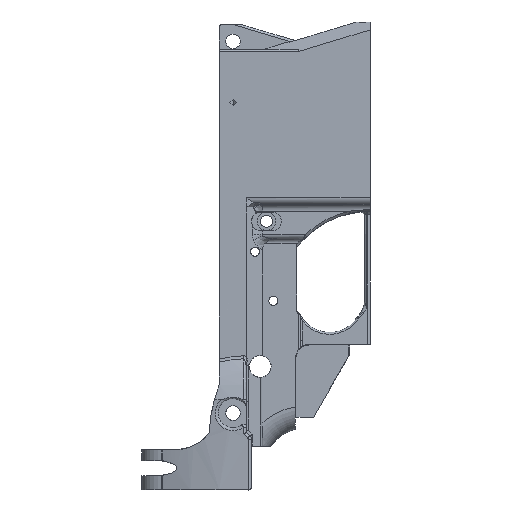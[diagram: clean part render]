
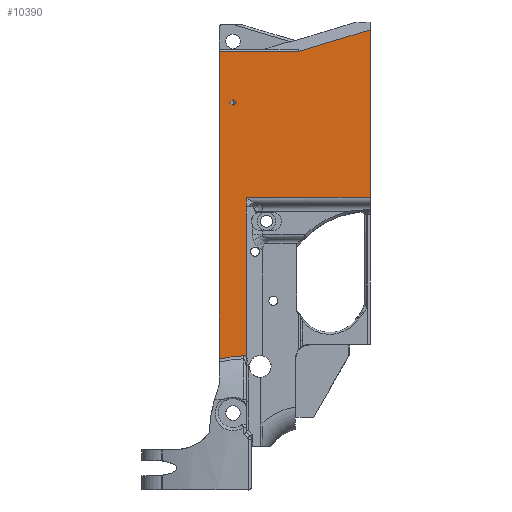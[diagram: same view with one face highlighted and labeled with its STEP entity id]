
A CAD part, left-side view. The second image highlights one B-rep face of the part: STEP entity #10390.
In plain terms, the highlighted planar face has unit normal (-1, 0, 0).
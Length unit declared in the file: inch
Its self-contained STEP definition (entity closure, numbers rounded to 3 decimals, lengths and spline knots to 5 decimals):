
#56=FACE_BOUND('',#1558,.T.);
#322=PLANE('',#11075);
#986=FACE_OUTER_BOUND('',#1557,.T.);
#1557=EDGE_LOOP('',(#7630,#7631,#7632,#7633,#7634,#7635,#7636,#7637,#7638,
#7639,#7640));
#1558=EDGE_LOOP('',(#7641,#7642,#7643,#7644));
#2303=B_SPLINE_CURVE_WITH_KNOTS('',3,(#20126,#20127,#20128,#20129),
 .UNSPECIFIED.,.F.,.F.,(4,4),(-1.31339,-0.24944),
 .UNSPECIFIED.);
#2304=B_SPLINE_CURVE_WITH_KNOTS('',3,(#20165,#20166,#20167,#20168),
 .UNSPECIFIED.,.F.,.F.,(4,4),(-0.14348,0.),
 .UNSPECIFIED.);
#2310=B_SPLINE_CURVE_WITH_KNOTS('',3,(#20292,#20293,#20294,#20295,#20296,
#20297),.UNSPECIFIED.,.F.,.F.,(4,1,1,4),(0.,0.33333,0.66667,
1.),.UNSPECIFIED.);
#2589=LINE('',#18092,#3299);
#2716=LINE('',#20286,#3426);
#2717=LINE('',#20288,#3427);
#2718=LINE('',#20290,#3428);
#2719=LINE('',#20299,#3429);
#2720=LINE('',#20301,#3430);
#2721=LINE('',#20303,#3431);
#2722=LINE('',#20304,#3432);
#2723=LINE('',#20307,#3433);
#2724=LINE('',#20309,#3434);
#2725=LINE('',#20311,#3435);
#2726=LINE('',#20312,#3436);
#3299=VECTOR('',#12008,6.06563);
#3426=VECTOR('',#12417,1.69849);
#3427=VECTOR('',#12418,0.3937);
#3428=VECTOR('',#12419,0.14801);
#3429=VECTOR('',#12420,2.12284);
#3430=VECTOR('',#12421,0.81541);
#3431=VECTOR('',#12422,1.28527);
#3432=VECTOR('',#12423,1.36014);
#3433=VECTOR('',#12424,0.3937);
#3434=VECTOR('',#12425,0.3937);
#3435=VECTOR('',#12426,0.3937);
#3436=VECTOR('',#12427,0.3937);
#4191=VERTEX_POINT('',#18077);
#4192=VERTEX_POINT('',#18091);
#4412=VERTEX_POINT('',#20053);
#4421=VERTEX_POINT('',#20124);
#4424=VERTEX_POINT('',#20285);
#4425=VERTEX_POINT('',#20287);
#4426=VERTEX_POINT('',#20289);
#4427=VERTEX_POINT('',#20291);
#4428=VERTEX_POINT('',#20298);
#4429=VERTEX_POINT('',#20300);
#4430=VERTEX_POINT('',#20302);
#4431=VERTEX_POINT('',#20305);
#4432=VERTEX_POINT('',#20306);
#4433=VERTEX_POINT('',#20308);
#4434=VERTEX_POINT('',#20310);
#5338=EDGE_CURVE('',#4191,#4192,#2589,.T.);
#5653=EDGE_CURVE('',#4421,#4191,#2303,.T.);
#5654=EDGE_CURVE('',#4412,#4421,#2304,.T.);
#5661=EDGE_CURVE('',#4424,#4412,#2716,.T.);
#5662=EDGE_CURVE('',#4424,#4425,#2717,.T.);
#5663=EDGE_CURVE('',#4425,#4426,#2718,.T.);
#5664=EDGE_CURVE('',#4426,#4427,#2310,.T.);
#5665=EDGE_CURVE('',#4427,#4428,#2719,.T.);
#5666=EDGE_CURVE('',#4428,#4429,#2720,.T.);
#5667=EDGE_CURVE('',#4429,#4430,#2721,.T.);
#5668=EDGE_CURVE('',#4192,#4430,#2722,.T.);
#5669=EDGE_CURVE('',#4431,#4432,#2723,.T.);
#5670=EDGE_CURVE('',#4432,#4433,#2724,.T.);
#5671=EDGE_CURVE('',#4433,#4434,#2725,.T.);
#5672=EDGE_CURVE('',#4434,#4431,#2726,.T.);
#7630=ORIENTED_EDGE('',*,*,#5654,.F.);
#7631=ORIENTED_EDGE('',*,*,#5661,.F.);
#7632=ORIENTED_EDGE('',*,*,#5662,.T.);
#7633=ORIENTED_EDGE('',*,*,#5663,.T.);
#7634=ORIENTED_EDGE('',*,*,#5664,.T.);
#7635=ORIENTED_EDGE('',*,*,#5665,.T.);
#7636=ORIENTED_EDGE('',*,*,#5666,.T.);
#7637=ORIENTED_EDGE('',*,*,#5667,.T.);
#7638=ORIENTED_EDGE('',*,*,#5668,.F.);
#7639=ORIENTED_EDGE('',*,*,#5338,.F.);
#7640=ORIENTED_EDGE('',*,*,#5653,.F.);
#7641=ORIENTED_EDGE('',*,*,#5669,.T.);
#7642=ORIENTED_EDGE('',*,*,#5670,.T.);
#7643=ORIENTED_EDGE('',*,*,#5671,.T.);
#7644=ORIENTED_EDGE('',*,*,#5672,.T.);
#10390=ADVANCED_FACE('',(#986,#56),#322,.F.);
#11075=AXIS2_PLACEMENT_3D('',#20284,#12415,#12416);
#12008=DIRECTION('',(0.,0.,1.));
#12415=DIRECTION('center_axis',(1.,0.,0.));
#12416=DIRECTION('ref_axis',(0.,0.,
-1.));
#12417=DIRECTION('',(0.,0.,-1.));
#12418=DIRECTION('',(0.,0.,1.));
#12419=DIRECTION('',(0.,0.,1.));
#12420=DIRECTION('',(0.,-1.,0.));
#12421=DIRECTION('',(0.,0.,1.));
#12422=DIRECTION('',(0.,0.957,-0.29));
#12423=DIRECTION('',(0.,-1.,0.));
#12424=DIRECTION('',(0.,-0.707,-0.707));
#12425=DIRECTION('',(0.,0.707,-0.707));
#12426=DIRECTION('',(0.,0.707,0.707));
#12427=DIRECTION('',(0.,-0.707,0.707));
#18077=CARTESIAN_POINT('',(-0.73097,1.33016,-2.19045));
#18091=CARTESIAN_POINT('',(-0.73097,1.33016,3.08063));
#18092=CARTESIAN_POINT('',(-0.73097,1.33016,-2.985));
#20053=CARTESIAN_POINT('',(-0.73097,0.86284,-2.15096));
#20124=CARTESIAN_POINT('',(-0.73097,0.91575,-2.13421));
#20126=CARTESIAN_POINT('Ctrl Pts',(-0.73097,0.91575,
-2.13421));
#20127=CARTESIAN_POINT('Ctrl Pts',(-0.73097,1.05528,
-2.13948));
#20128=CARTESIAN_POINT('Ctrl Pts',(-0.73097,1.19434,
-2.15806));
#20129=CARTESIAN_POINT('Ctrl Pts',(-0.73097,1.33016,
-2.19045));
#20165=CARTESIAN_POINT('Ctrl Pts',(-0.73097,0.86288,
-2.15105));
#20166=CARTESIAN_POINT('Ctrl Pts',(-0.73097,0.87842,
-2.14036));
#20167=CARTESIAN_POINT('Ctrl Pts',(-0.73097,0.89693,
-2.1335));
#20168=CARTESIAN_POINT('Ctrl Pts',(-0.73097,0.91575,
-2.13421));
#20284=CARTESIAN_POINT('Origin',(-0.73097,0.68,-3.68485));
#20285=CARTESIAN_POINT('',(-0.73097,0.86284,0.4168));
#20286=CARTESIAN_POINT('',(-0.73097,0.86284,-2.50014));
#20287=CARTESIAN_POINT('',(-0.73095,0.86283,0.4836));
#20288=CARTESIAN_POINT('',(-0.73097,0.86284,-3.96143));
#20289=CARTESIAN_POINT('',(-0.7309,0.86284,0.56481));
#20290=CARTESIAN_POINT('',(-0.73097,0.86284,0.4168));
#20291=CARTESIAN_POINT('',(-0.73097,0.86284,0.57169));
#20292=CARTESIAN_POINT('Ctrl Pts',(-0.7309,0.86284,
0.56481));
#20293=CARTESIAN_POINT('Ctrl Pts',(-0.7309,0.86284,
0.56557));
#20294=CARTESIAN_POINT('Ctrl Pts',(-0.731,0.86284,
0.5671));
#20295=CARTESIAN_POINT('Ctrl Pts',(-0.73096,0.86284,
0.56939));
#20296=CARTESIAN_POINT('Ctrl Pts',(-0.73097,0.86284,
0.57092));
#20297=CARTESIAN_POINT('Ctrl Pts',(-0.73097,0.86284,
0.57169));
#20298=CARTESIAN_POINT('',(-0.73097,-1.26,0.57169));
#20299=CARTESIAN_POINT('',(-0.73097,0.86284,0.57169));
#20300=CARTESIAN_POINT('',(-0.73097,-1.26,3.45341));
#20301=CARTESIAN_POINT('',(-0.73097,-1.26,2.63799));
#20302=CARTESIAN_POINT('',(-0.73097,-0.02998,3.08063));
#20303=CARTESIAN_POINT('',(-0.73097,-1.26,3.45341));
#20304=CARTESIAN_POINT('',(-0.73097,1.33016,3.08063));
#20305=CARTESIAN_POINT('',(-0.73097,1.0895,2.26515));
#20306=CARTESIAN_POINT('',(-0.73097,1.03435,2.21));
#20307=CARTESIAN_POINT('',(-0.73097,-0.50038,0.67528));
#20308=CARTESIAN_POINT('',(-0.73097,1.0895,2.15485));
#20309=CARTESIAN_POINT('',(-0.73097,2.41947,0.82487));
#20310=CARTESIAN_POINT('',(-0.73097,1.14465,2.21));
#20311=CARTESIAN_POINT('',(-0.73097,-0.4728,0.59255));
#20312=CARTESIAN_POINT('',(-0.73097,2.5022,0.85245));
